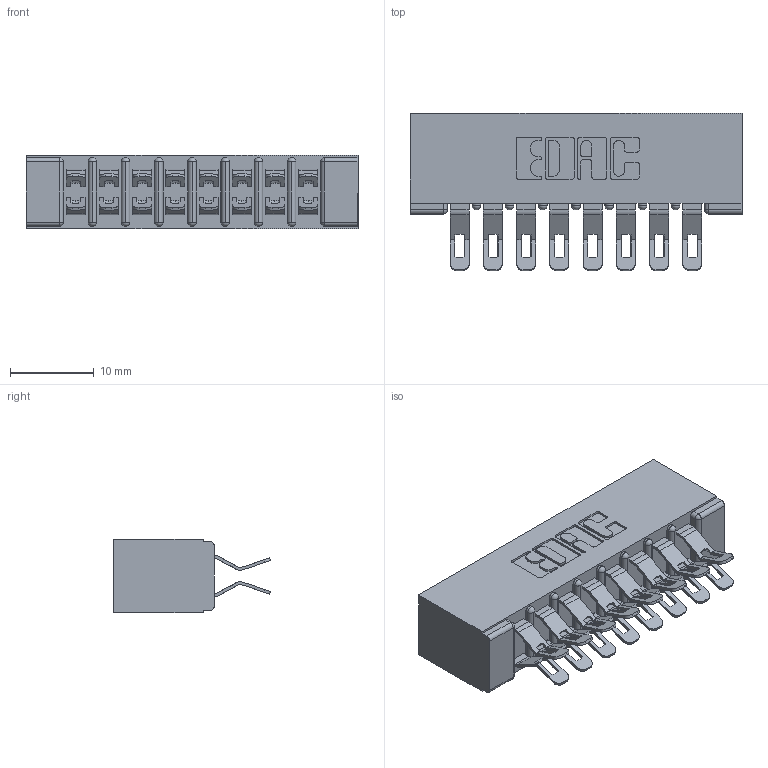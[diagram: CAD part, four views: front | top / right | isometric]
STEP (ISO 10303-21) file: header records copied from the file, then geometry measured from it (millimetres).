
FILE_DESCRIPTION (( 'STEP AP203' ), '1' );
FILE_NAME ('307-016-455-201.STEP', '2020-09-28T17:27:14', ( '' ), ( '' ), 'SwSTEP 2.0', 'SolidWorks 2020', '' );
FILE_SCHEMA (( 'CONFIG_CONTROL_DESIGN' ));
Length unit declared in the file: inch
Products named in the file (3): 307-016-455-201; 307 Part_No Mounting Lugs; 307-290-001_555
Assembly tree (17 placements, depth 2):
  307-016-455-201
    307 Part_No Mounting Lugs
    307-290-001_555  x16
Bounding box: 39.57 x 18.75 x 8.71 mm (x, y, z)
Volume: 2870.9 mm3; surface area: 5074.5 mm2
Topology: 17 solids, 17 shells, 1095 faces, 3195 edges, 2082 vertices
Faces by surface type: plane 610, cylinder 467, sphere 18
Entity records: 11565 total; most frequent: CARTESIAN_POINT 1904, DIRECTION 1886, ORIENTED_EDGE 1884, EDGE_CURVE 942, VECTOR 698, LINE 698, VERTEX_POINT 612, AXIS2_PLACEMENT_3D 594
